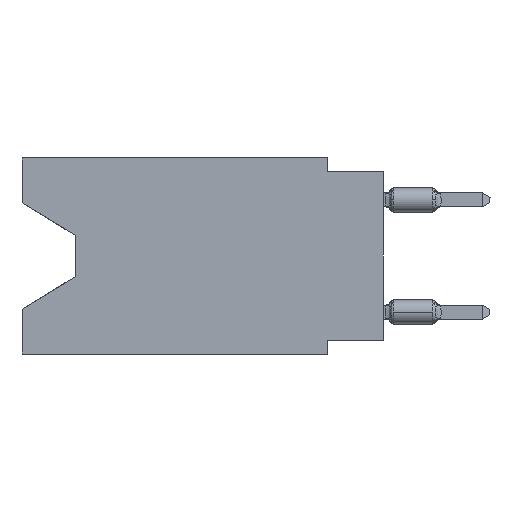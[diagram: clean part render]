
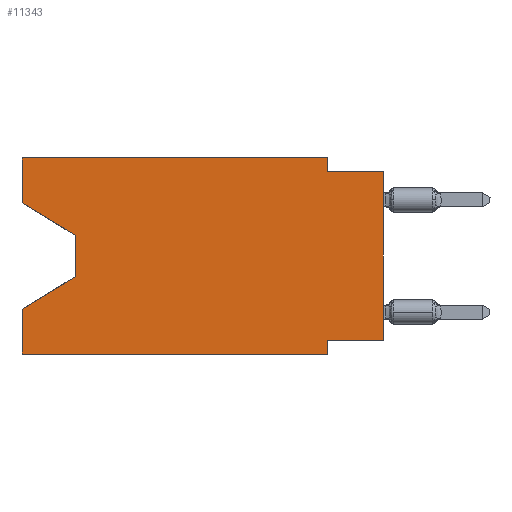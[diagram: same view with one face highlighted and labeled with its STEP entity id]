
A CAD part, left-side view. The second image highlights one B-rep face of the part: STEP entity #11343.
In plain terms, the highlighted planar face has unit normal (-1, 0, 0).
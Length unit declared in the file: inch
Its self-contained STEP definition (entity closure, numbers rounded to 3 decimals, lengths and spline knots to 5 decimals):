
#390 = VECTOR ( 'NONE', #38671, 39.37008 ) ;
#1576 = CARTESIAN_POINT ( 'NONE',  ( 0., 0.1, 0. ) ) ;
#2545 = CARTESIAN_POINT ( 'NONE',  ( 0., 0.1, -0.025 ) ) ;
#2789 = CARTESIAN_POINT ( 'NONE',  ( 0., 0.1, -0.35 ) ) ;
#3116 = EDGE_CURVE ( 'NONE', #5107, #20590, #19525, .T. ) ;
#4478 = CARTESIAN_POINT ( 'NONE',  ( 0., 0.645, -0.26975 ) ) ;
#4818 = VECTOR ( 'NONE', #35335, 39.37008 ) ;
#5107 = VERTEX_POINT ( 'NONE', #18708 ) ;
#5224 = DIRECTION ( 'NONE',  ( 1., 0., 0. ) ) ;
#5616 = CARTESIAN_POINT ( 'NONE',  ( 0., 0.55, -0.138 ) ) ;
#6871 = ORIENTED_EDGE ( 'NONE', *, *, #39276, .T. ) ;
#8179 = VECTOR ( 'NONE', #29050, 39.37008 ) ;
#8613 = ORIENTED_EDGE ( 'NONE', *, *, #25818, .F. ) ;
#9152 = ORIENTED_EDGE ( 'NONE', *, *, #38894, .F. ) ;
#9310 = DIRECTION ( 'NONE',  ( 0., 0., -1. ) ) ;
#9798 = EDGE_CURVE ( 'NONE', #46629, #29231, #12792, .T. ) ;
#10869 = DIRECTION ( 'NONE',  ( 0., 0.855, -0.519 ) ) ;
#10927 = LINE ( 'NONE', #26115, #8179 ) ;
#11343 = ADVANCED_FACE ( 'NONE', ( #17426 ), #24306, .F. ) ;
#11409 = EDGE_CURVE ( 'NONE', #21417, #20238, #43150, .T. ) ;
#11568 = VECTOR ( 'NONE', #20903, 39.37008 ) ;
#12792 = LINE ( 'NONE', #1576, #4818 ) ;
#13309 = LINE ( 'NONE', #39738, #11568 ) ;
#13343 = VERTEX_POINT ( 'NONE', #24136 ) ;
#13428 = ORIENTED_EDGE ( 'NONE', *, *, #3116, .T. ) ;
#13435 = LINE ( 'NONE', #24460, #390 ) ;
#13692 = ORIENTED_EDGE ( 'NONE', *, *, #42743, .T. ) ;
#13741 = VECTOR ( 'NONE', #17198, 39.37008 ) ;
#13800 = VECTOR ( 'NONE', #9310, 39.37008 ) ;
#13809 = EDGE_CURVE ( 'NONE', #32755, #20238, #47966, .T. ) ;
#13923 = LINE ( 'NONE', #47478, #36045 ) ;
#14397 = CARTESIAN_POINT ( 'NONE',  ( 0., 0.645, -0.35 ) ) ;
#14445 = VECTOR ( 'NONE', #10869, 39.37008 ) ;
#15400 = VERTEX_POINT ( 'NONE', #47556 ) ;
#15412 = CARTESIAN_POINT ( 'NONE',  ( 0., 0.645, 0. ) ) ;
#16172 = DIRECTION ( 'NONE',  ( 0., -1., 0. ) ) ;
#16550 = CARTESIAN_POINT ( 'NONE',  ( 0., 0.1, 0. ) ) ;
#17198 = DIRECTION ( 'NONE',  ( 0., 0., -1. ) ) ;
#17227 = CARTESIAN_POINT ( 'NONE',  ( 0., 0., -0.325 ) ) ;
#17426 = FACE_OUTER_BOUND ( 'NONE', #35191, .T. ) ;
#17511 = ORIENTED_EDGE ( 'NONE', *, *, #13809, .T. ) ;
#18294 = EDGE_CURVE ( 'NONE', #32755, #28307, #13923, .T. ) ;
#18708 = CARTESIAN_POINT ( 'NONE',  ( 0., 0.645, -0.08025 ) ) ;
#19422 = EDGE_CURVE ( 'NONE', #29231, #46225, #42611, .T. ) ;
#19525 = LINE ( 'NONE', #37885, #47857 ) ;
#20023 = AXIS2_PLACEMENT_3D ( 'NONE', #31426, #5224, #43633 ) ;
#20238 = VERTEX_POINT ( 'NONE', #2789 ) ;
#20572 = VECTOR ( 'NONE', #30381, 39.37008 ) ;
#20590 = VERTEX_POINT ( 'NONE', #33800 ) ;
#20903 = DIRECTION ( 'NONE',  ( 0., 0., 1. ) ) ;
#21417 = VERTEX_POINT ( 'NONE', #39586 ) ;
#21899 = ORIENTED_EDGE ( 'NONE', *, *, #18294, .F. ) ;
#24136 = CARTESIAN_POINT ( 'NONE',  ( 0., 0.55, -0.212 ) ) ;
#24306 = PLANE ( 'NONE',  #20023 ) ;
#24460 = CARTESIAN_POINT ( 'NONE',  ( 0., 0.645, 0. ) ) ;
#25661 = ORIENTED_EDGE ( 'NONE', *, *, #27101, .F. ) ;
#25818 = EDGE_CURVE ( 'NONE', #5107, #15400, #34031, .T. ) ;
#26115 = CARTESIAN_POINT ( 'NONE',  ( 0., 0., -0.325 ) ) ;
#26282 = VERTEX_POINT ( 'NONE', #17227 ) ;
#27101 = EDGE_CURVE ( 'NONE', #15400, #46629, #13435, .T. ) ;
#27241 = CARTESIAN_POINT ( 'NONE',  ( 0., 0., -0.025 ) ) ;
#28307 = VERTEX_POINT ( 'NONE', #4478 ) ;
#29050 = DIRECTION ( 'NONE',  ( 0., 1., 0. ) ) ;
#29231 = VERTEX_POINT ( 'NONE', #2545 ) ;
#30381 = DIRECTION ( 'NONE',  ( 0., 0., 1. ) ) ;
#31426 = CARTESIAN_POINT ( 'NONE',  ( 0., 0.645, 0. ) ) ;
#32125 = CARTESIAN_POINT ( 'NONE',  ( 0., 0.645, -0.35 ) ) ;
#32691 = LINE ( 'NONE', #44164, #14445 ) ;
#32755 = VERTEX_POINT ( 'NONE', #32125 ) ;
#33182 = EDGE_CURVE ( 'NONE', #20590, #13343, #42855, .T. ) ;
#33800 = CARTESIAN_POINT ( 'NONE',  ( 0., 0.55, -0.138 ) ) ;
#34031 = LINE ( 'NONE', #15412, #20572 ) ;
#34790 = CARTESIAN_POINT ( 'NONE',  ( 0., 0., -0.025 ) ) ;
#34888 = ORIENTED_EDGE ( 'NONE', *, *, #33182, .T. ) ;
#35191 = EDGE_LOOP ( 'NONE', ( #13428, #34888, #6871, #21899, #17511, #44921, #9152, #13692, #42471, #36036, #25661, #8613 ) ) ;
#35335 = DIRECTION ( 'NONE',  ( 0., 0., -1. ) ) ;
#35565 = CARTESIAN_POINT ( 'NONE',  ( 0., 0.1, -0.35 ) ) ;
#36036 = ORIENTED_EDGE ( 'NONE', *, *, #9798, .F. ) ;
#36045 = VECTOR ( 'NONE', #43554, 39.37008 ) ;
#37885 = CARTESIAN_POINT ( 'NONE',  ( 0., 0.645, -0.08025 ) ) ;
#38671 = DIRECTION ( 'NONE',  ( 0., -1., 0. ) ) ;
#38894 = EDGE_CURVE ( 'NONE', #26282, #21417, #10927, .T. ) ;
#39276 = EDGE_CURVE ( 'NONE', #13343, #28307, #32691, .T. ) ;
#39586 = CARTESIAN_POINT ( 'NONE',  ( 0., 0.1, -0.325 ) ) ;
#39738 = CARTESIAN_POINT ( 'NONE',  ( 0., 0., 0. ) ) ;
#40619 = DIRECTION ( 'NONE',  ( 0., -1., 0. ) ) ;
#42471 = ORIENTED_EDGE ( 'NONE', *, *, #19422, .F. ) ;
#42534 = DIRECTION ( 'NONE',  ( 0., -0.855, -0.519 ) ) ;
#42611 = LINE ( 'NONE', #34790, #46304 ) ;
#42743 = EDGE_CURVE ( 'NONE', #26282, #46225, #13309, .T. ) ;
#42855 = LINE ( 'NONE', #5616, #13800 ) ;
#43150 = LINE ( 'NONE', #35565, #13741 ) ;
#43554 = DIRECTION ( 'NONE',  ( 0., 0., 1. ) ) ;
#43633 = DIRECTION ( 'NONE',  ( 0., 0., -1. ) ) ;
#44164 = CARTESIAN_POINT ( 'NONE',  ( 0., 0.55, -0.212 ) ) ;
#44921 = ORIENTED_EDGE ( 'NONE', *, *, #11409, .F. ) ;
#46225 = VERTEX_POINT ( 'NONE', #27241 ) ;
#46304 = VECTOR ( 'NONE', #16172, 39.37008 ) ;
#46629 = VERTEX_POINT ( 'NONE', #16550 ) ;
#47478 = CARTESIAN_POINT ( 'NONE',  ( 0., 0.645, 0. ) ) ;
#47556 = CARTESIAN_POINT ( 'NONE',  ( 0., 0.645, 0. ) ) ;
#47857 = VECTOR ( 'NONE', #42534, 39.37008 ) ;
#47966 = LINE ( 'NONE', #14397, #48362 ) ;
#48362 = VECTOR ( 'NONE', #40619, 39.37008 ) ;
